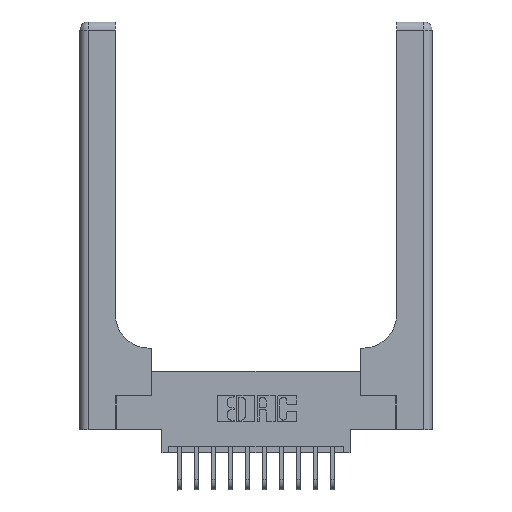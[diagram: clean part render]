
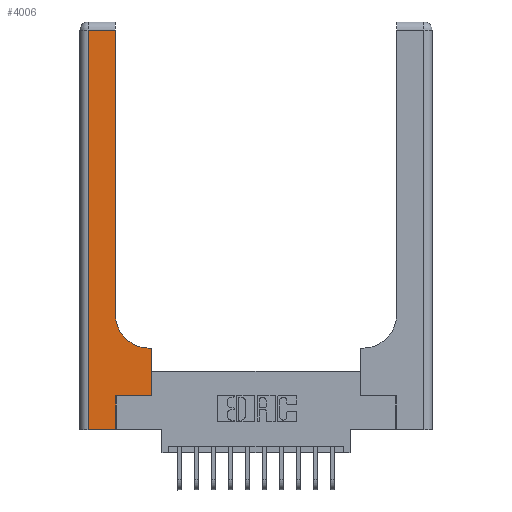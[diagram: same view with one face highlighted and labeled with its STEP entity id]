
A CAD part, top view. The second image highlights one B-rep face of the part: STEP entity #4006.
In plain terms, the highlighted planar face has unit normal (0, 0, 1).
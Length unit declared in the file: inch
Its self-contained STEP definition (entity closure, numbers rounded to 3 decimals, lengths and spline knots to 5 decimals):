
#78 = VECTOR ( 'NONE', #12151, 39.37008 ) ;
#257 = CARTESIAN_POINT ( 'NONE',  ( 0.06, 0., 0.37 ) ) ;
#689 = VECTOR ( 'NONE', #16884, 39.37008 ) ;
#1152 = EDGE_LOOP ( 'NONE', ( #13034, #16489, #5007, #6169, #13049, #4636, #15089, #4448, #1987 ) ) ;
#1364 = DIRECTION ( 'NONE',  ( -1., 0., 0. ) ) ;
#1632 = VECTOR ( 'NONE', #12796, 39.37008 ) ;
#1836 = LINE ( 'NONE', #9464, #14158 ) ;
#1858 = EDGE_CURVE ( 'NONE', #16412, #5721, #9480, .T. ) ;
#1987 = ORIENTED_EDGE ( 'NONE', *, *, #1858, .T. ) ;
#2319 = CARTESIAN_POINT ( 'NONE',  ( 0.26, 2.94, 0.37 ) ) ;
#2423 = DIRECTION ( 'NONE',  ( 0., 0., -1. ) ) ;
#2760 = CARTESIAN_POINT ( 'NONE',  ( 0.265, 0.25, 0.37 ) ) ;
#3146 = VERTEX_POINT ( 'NONE', #11554 ) ;
#3483 = DIRECTION ( 'NONE',  ( -1., 0., 0. ) ) ;
#3789 = DIRECTION ( 'NONE',  ( 1., 0., 0. ) ) ;
#3826 = CARTESIAN_POINT ( 'NONE',  ( 0.06, 3., 0.37 ) ) ;
#4006 = ADVANCED_FACE ( 'NONE', ( #12028 ), #8686, .F. ) ;
#4448 = ORIENTED_EDGE ( 'NONE', *, *, #17840, .T. ) ;
#4636 = ORIENTED_EDGE ( 'NONE', *, *, #5284, .T. ) ;
#5007 = ORIENTED_EDGE ( 'NONE', *, *, #17141, .T. ) ;
#5203 = VECTOR ( 'NONE', #11137, 39.37008 ) ;
#5212 = VERTEX_POINT ( 'NONE', #8804 ) ;
#5270 = VERTEX_POINT ( 'NONE', #257 ) ;
#5284 = EDGE_CURVE ( 'NONE', #13880, #8215, #7878, .T. ) ;
#5326 = DIRECTION ( 'NONE',  ( -1., 0., 0. ) ) ;
#5721 = VERTEX_POINT ( 'NONE', #8335 ) ;
#5954 = LINE ( 'NONE', #9368, #78 ) ;
#6169 = ORIENTED_EDGE ( 'NONE', *, *, #11670, .T. ) ;
#6326 = DIRECTION ( 'NONE',  ( 0., -1., 0. ) ) ;
#6567 = EDGE_CURVE ( 'NONE', #17771, #17408, #1836, .T. ) ;
#7000 = LINE ( 'NONE', #10894, #10263 ) ;
#7062 = CARTESIAN_POINT ( 'NONE',  ( 0.265, 0., 0.37 ) ) ;
#7878 = LINE ( 'NONE', #12911, #1632 ) ;
#8215 = VERTEX_POINT ( 'NONE', #10883 ) ;
#8335 = CARTESIAN_POINT ( 'NONE',  ( 0.26, 0.85, 0.37 ) ) ;
#8686 = PLANE ( 'NONE',  #12714 ) ;
#8804 = CARTESIAN_POINT ( 'NONE',  ( 0.265, 0., 0.37 ) ) ;
#8844 = AXIS2_PLACEMENT_3D ( 'NONE', #9171, #2423, #3789 ) ;
#8892 = LINE ( 'NONE', #15161, #5203 ) ;
#8925 = DIRECTION ( 'NONE',  ( 0., 0., -1. ) ) ;
#9171 = CARTESIAN_POINT ( 'NONE',  ( 0.51, 0.85, 0.37 ) ) ;
#9368 = CARTESIAN_POINT ( 'NONE',  ( 0.528, 0.25, 0.37 ) ) ;
#9464 = CARTESIAN_POINT ( 'NONE',  ( 0., 2.94, 0.37 ) ) ;
#9480 = CIRCLE ( 'NONE', #8844, 0.25 ) ;
#9970 = LINE ( 'NONE', #7062, #14083 ) ;
#10101 = CARTESIAN_POINT ( 'NONE',  ( 0., 3., 0.37 ) ) ;
#10263 = VECTOR ( 'NONE', #5326, 39.37008 ) ;
#10844 = LINE ( 'NONE', #3826, #11082 ) ;
#10883 = CARTESIAN_POINT ( 'NONE',  ( 0.528, 0.25, 0.37 ) ) ;
#10894 = CARTESIAN_POINT ( 'NONE',  ( 0.26, 0.6, 0.37 ) ) ;
#11082 = VECTOR ( 'NONE', #6326, 39.37008 ) ;
#11137 = DIRECTION ( 'NONE',  ( 0., 1., 0. ) ) ;
#11554 = CARTESIAN_POINT ( 'NONE',  ( 0.528, 0.6, 0.37 ) ) ;
#11572 = CARTESIAN_POINT ( 'NONE',  ( 0.06, 2.94, 0.37 ) ) ;
#11670 = EDGE_CURVE ( 'NONE', #5270, #5212, #14970, .T. ) ;
#12028 = FACE_OUTER_BOUND ( 'NONE', #1152, .T. ) ;
#12151 = DIRECTION ( 'NONE',  ( 0., 1., 0. ) ) ;
#12376 = EDGE_CURVE ( 'NONE', #5721, #17771, #8892, .T. ) ;
#12382 = DIRECTION ( 'NONE',  ( 0., 1., 0. ) ) ;
#12714 = AXIS2_PLACEMENT_3D ( 'NONE', #10101, #8925, #3483 ) ;
#12796 = DIRECTION ( 'NONE',  ( 1., 0., 0. ) ) ;
#12911 = CARTESIAN_POINT ( 'NONE',  ( 0.265, 0.25, 0.37 ) ) ;
#12964 = CARTESIAN_POINT ( 'NONE',  ( 0., 0., 0.37 ) ) ;
#13034 = ORIENTED_EDGE ( 'NONE', *, *, #12376, .T. ) ;
#13049 = ORIENTED_EDGE ( 'NONE', *, *, #13723, .T. ) ;
#13723 = EDGE_CURVE ( 'NONE', #5212, #13880, #9970, .T. ) ;
#13880 = VERTEX_POINT ( 'NONE', #2760 ) ;
#14083 = VECTOR ( 'NONE', #12382, 39.37008 ) ;
#14158 = VECTOR ( 'NONE', #1364, 39.37008 ) ;
#14970 = LINE ( 'NONE', #12964, #689 ) ;
#15089 = ORIENTED_EDGE ( 'NONE', *, *, #17794, .T. ) ;
#15161 = CARTESIAN_POINT ( 'NONE',  ( 0.26, 3., 0.37 ) ) ;
#16412 = VERTEX_POINT ( 'NONE', #17357 ) ;
#16489 = ORIENTED_EDGE ( 'NONE', *, *, #6567, .T. ) ;
#16884 = DIRECTION ( 'NONE',  ( 1., 0., 0. ) ) ;
#17141 = EDGE_CURVE ( 'NONE', #17408, #5270, #10844, .T. ) ;
#17357 = CARTESIAN_POINT ( 'NONE',  ( 0.51, 0.6, 0.37 ) ) ;
#17408 = VERTEX_POINT ( 'NONE', #11572 ) ;
#17771 = VERTEX_POINT ( 'NONE', #2319 ) ;
#17794 = EDGE_CURVE ( 'NONE', #8215, #3146, #5954, .T. ) ;
#17840 = EDGE_CURVE ( 'NONE', #3146, #16412, #7000, .T. ) ;
